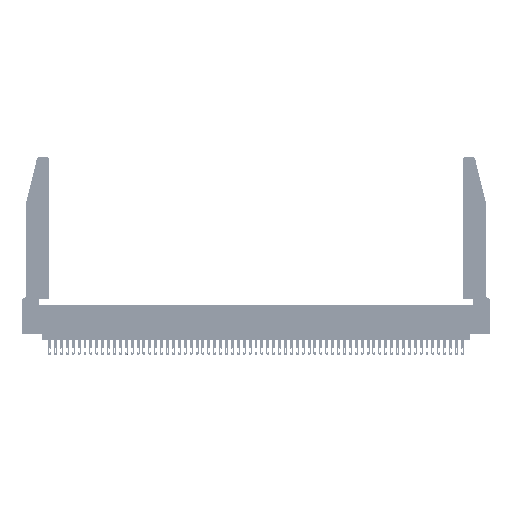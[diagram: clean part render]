
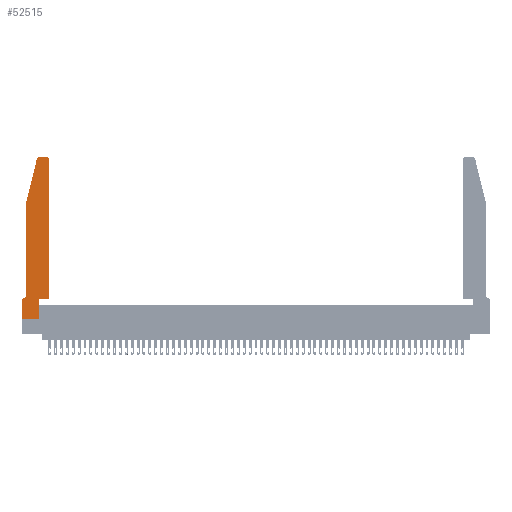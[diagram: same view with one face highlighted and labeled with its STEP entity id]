
A CAD part, top view. The second image highlights one B-rep face of the part: STEP entity #52515.
In plain terms, the highlighted planar face has unit normal (0, 0, 1).
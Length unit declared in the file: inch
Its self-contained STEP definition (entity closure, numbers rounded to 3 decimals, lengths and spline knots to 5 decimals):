
#226 = CARTESIAN_POINT ( 'NONE',  ( 0.0755, 2., 0.37 ) ) ;
#576 = EDGE_CURVE ( 'NONE', #30748, #18851, #41147, .T. ) ;
#718 = LINE ( 'NONE', #26507, #32840 ) ;
#1125 = DIRECTION ( 'NONE',  ( 1., 0., 0. ) ) ;
#3038 = CARTESIAN_POINT ( 'NONE',  ( 0., 0.35, 0.37 ) ) ;
#4143 = DIRECTION ( 'NONE',  ( 0., -1., 0. ) ) ;
#5221 = AXIS2_PLACEMENT_3D ( 'NONE', #51670, #29842, #34268 ) ;
#5655 = DIRECTION ( 'NONE',  ( 0., 1., 0. ) ) ;
#6487 = DIRECTION ( 'NONE',  ( -0.239, -0.971, 0. ) ) ;
#6604 = VECTOR ( 'NONE', #6487, 39.37008 ) ;
#6764 = CARTESIAN_POINT ( 'NONE',  ( 0.284, 2.75, 0.37 ) ) ;
#8374 = DIRECTION ( 'NONE',  ( 0., 1., 0. ) ) ;
#8848 = CARTESIAN_POINT ( 'NONE',  ( 0.4205, 2.75, 0.37 ) ) ;
#9397 = CARTESIAN_POINT ( 'NONE',  ( 0.4505, 0.35, 0.37 ) ) ;
#9897 = LINE ( 'NONE', #36895, #14660 ) ;
#10339 = DIRECTION ( 'NONE',  ( -1., 0., 0. ) ) ;
#10479 = VERTEX_POINT ( 'NONE', #226 ) ;
#10501 = LINE ( 'NONE', #42448, #13964 ) ;
#12745 = CARTESIAN_POINT ( 'NONE',  ( 0.0755, 2., 0.37 ) ) ;
#13517 = VERTEX_POINT ( 'NONE', #6764 ) ;
#13951 = EDGE_CURVE ( 'NONE', #18851, #16450, #26975, .T. ) ;
#13964 = VECTOR ( 'NONE', #33268, 39.37008 ) ;
#14003 = CARTESIAN_POINT ( 'NONE',  ( 0.284, 2.72, 0.37 ) ) ;
#14508 = CARTESIAN_POINT ( 'NONE',  ( 0., 0., 0.37 ) ) ;
#14602 = VERTEX_POINT ( 'NONE', #14508 ) ;
#14660 = VECTOR ( 'NONE', #10339, 39.37008 ) ;
#15905 = ORIENTED_EDGE ( 'NONE', *, *, #17103, .T. ) ;
#15921 = FACE_OUTER_BOUND ( 'NONE', #51084, .T. ) ;
#16450 = VERTEX_POINT ( 'NONE', #55902 ) ;
#16489 = ORIENTED_EDGE ( 'NONE', *, *, #45321, .T. ) ;
#16892 = VERTEX_POINT ( 'NONE', #28303 ) ;
#17103 = EDGE_CURVE ( 'NONE', #33877, #13517, #10501, .T. ) ;
#17626 = DIRECTION ( 'NONE',  ( 1., 0., 0. ) ) ;
#18584 = DIRECTION ( 'NONE',  ( 1., 0., 0. ) ) ;
#18851 = VERTEX_POINT ( 'NONE', #42649 ) ;
#19856 = CARTESIAN_POINT ( 'NONE',  ( 0.0755, 2., 0.37 ) ) ;
#20776 = LINE ( 'NONE', #12745, #55700 ) ;
#21788 = EDGE_CURVE ( 'NONE', #31913, #33877, #22995, .T. ) ;
#22226 = EDGE_CURVE ( 'NONE', #52866, #14602, #39295, .T. ) ;
#22379 = DIRECTION ( 'NONE',  ( 0., 0., 1. ) ) ;
#22546 = ORIENTED_EDGE ( 'NONE', *, *, #44567, .T. ) ;
#22633 = CARTESIAN_POINT ( 'NONE',  ( 0.4505, 0.35, 0.37 ) ) ;
#22995 = CIRCLE ( 'NONE', #53683, 0.03 ) ;
#23276 = EDGE_CURVE ( 'NONE', #30683, #52866, #9897, .T. ) ;
#24157 = CARTESIAN_POINT ( 'NONE',  ( 0., 0.35, 0.37 ) ) ;
#24396 = ORIENTED_EDGE ( 'NONE', *, *, #576, .T. ) ;
#24911 = AXIS2_PLACEMENT_3D ( 'NONE', #3038, #55236, #46423 ) ;
#26013 = CIRCLE ( 'NONE', #51795, 0.03 ) ;
#26507 = CARTESIAN_POINT ( 'NONE',  ( 0., 0., 0.37 ) ) ;
#26975 = LINE ( 'NONE', #9397, #46776 ) ;
#27653 = VECTOR ( 'NONE', #34147, 39.37008 ) ;
#28303 = CARTESIAN_POINT ( 'NONE',  ( 0.0755, 0.42, 0.37 ) ) ;
#29842 = DIRECTION ( 'NONE',  ( 0., 0., -1. ) ) ;
#30683 = VERTEX_POINT ( 'NONE', #37601 ) ;
#30748 = VERTEX_POINT ( 'NONE', #46753 ) ;
#31353 = EDGE_CURVE ( 'NONE', #10479, #16892, #20776, .T. ) ;
#31529 = DIRECTION ( 'NONE',  ( 0., 0., 1. ) ) ;
#31635 = ORIENTED_EDGE ( 'NONE', *, *, #23276, .T. ) ;
#31913 = VERTEX_POINT ( 'NONE', #42678 ) ;
#32477 = LINE ( 'NONE', #22633, #35902 ) ;
#32840 = VECTOR ( 'NONE', #35879, 39.37008 ) ;
#33268 = DIRECTION ( 'NONE',  ( -1., 0., 0. ) ) ;
#33877 = VERTEX_POINT ( 'NONE', #8848 ) ;
#34000 = EDGE_CURVE ( 'NONE', #13517, #55807, #26013, .T. ) ;
#34147 = DIRECTION ( 'NONE',  ( 0., -1., 0. ) ) ;
#34268 = DIRECTION ( 'NONE',  ( -1., 0., 0. ) ) ;
#34375 = ORIENTED_EDGE ( 'NONE', *, *, #50514, .T. ) ;
#34562 = ORIENTED_EDGE ( 'NONE', *, *, #21788, .T. ) ;
#34718 = CARTESIAN_POINT ( 'NONE',  ( 0., 0., 0.37 ) ) ;
#35261 = ORIENTED_EDGE ( 'NONE', *, *, #31353, .T. ) ;
#35879 = DIRECTION ( 'NONE',  ( 1., 0., 0. ) ) ;
#35902 = VECTOR ( 'NONE', #5655, 39.37008 ) ;
#36872 = ORIENTED_EDGE ( 'NONE', *, *, #51586, .T. ) ;
#36895 = CARTESIAN_POINT ( 'NONE',  ( 0.0755, 0.35, 0.37 ) ) ;
#37601 = CARTESIAN_POINT ( 'NONE',  ( 0.0055, 0.35, 0.37 ) ) ;
#39295 = LINE ( 'NONE', #34718, #27653 ) ;
#39622 = ORIENTED_EDGE ( 'NONE', *, *, #34000, .T. ) ;
#41147 = LINE ( 'NONE', #52527, #55536 ) ;
#42188 = ORIENTED_EDGE ( 'NONE', *, *, #13951, .T. ) ;
#42448 = CARTESIAN_POINT ( 'NONE',  ( 0.2605, 2.75, 0.37 ) ) ;
#42649 = CARTESIAN_POINT ( 'NONE',  ( 0.2865, 0.35, 0.37 ) ) ;
#42678 = CARTESIAN_POINT ( 'NONE',  ( 0.4505, 2.72, 0.37 ) ) ;
#44229 = LINE ( 'NONE', #19856, #6604 ) ;
#44567 = EDGE_CURVE ( 'NONE', #16892, #30683, #50802, .T. ) ;
#45321 = EDGE_CURVE ( 'NONE', #14602, #30748, #718, .T. ) ;
#46423 = DIRECTION ( 'NONE',  ( 1., 0., 0. ) ) ;
#46753 = CARTESIAN_POINT ( 'NONE',  ( 0.2865, 0., 0.37 ) ) ;
#46776 = VECTOR ( 'NONE', #17626, 39.37008 ) ;
#49659 = CARTESIAN_POINT ( 'NONE',  ( 0.4205, 2.72, 0.37 ) ) ;
#50101 = ORIENTED_EDGE ( 'NONE', *, *, #22226, .T. ) ;
#50514 = EDGE_CURVE ( 'NONE', #55807, #10479, #44229, .T. ) ;
#50802 = CIRCLE ( 'NONE', #5221, 0.07 ) ;
#51084 = EDGE_LOOP ( 'NONE', ( #15905, #39622, #34375, #35261, #22546, #31635, #50101, #16489, #24396, #42188, #36872, #34562 ) ) ;
#51420 = PLANE ( 'NONE',  #24911 ) ;
#51586 = EDGE_CURVE ( 'NONE', #16450, #31913, #32477, .T. ) ;
#51670 = CARTESIAN_POINT ( 'NONE',  ( 0.0055, 0.42, 0.37 ) ) ;
#51795 = AXIS2_PLACEMENT_3D ( 'NONE', #14003, #22379, #18584 ) ;
#52515 = ADVANCED_FACE ( 'NONE', ( #15921 ), #51420, .T. ) ;
#52527 = CARTESIAN_POINT ( 'NONE',  ( 0.2865, 0.35, 0.37 ) ) ;
#52866 = VERTEX_POINT ( 'NONE', #24157 ) ;
#53259 = CARTESIAN_POINT ( 'NONE',  ( 0.25487, 2.72718, 0.37 ) ) ;
#53683 = AXIS2_PLACEMENT_3D ( 'NONE', #49659, #31529, #1125 ) ;
#55236 = DIRECTION ( 'NONE',  ( 0., 0., 1. ) ) ;
#55536 = VECTOR ( 'NONE', #8374, 39.37008 ) ;
#55700 = VECTOR ( 'NONE', #4143, 39.37008 ) ;
#55807 = VERTEX_POINT ( 'NONE', #53259 ) ;
#55902 = CARTESIAN_POINT ( 'NONE',  ( 0.4505, 0.35, 0.37 ) ) ;
